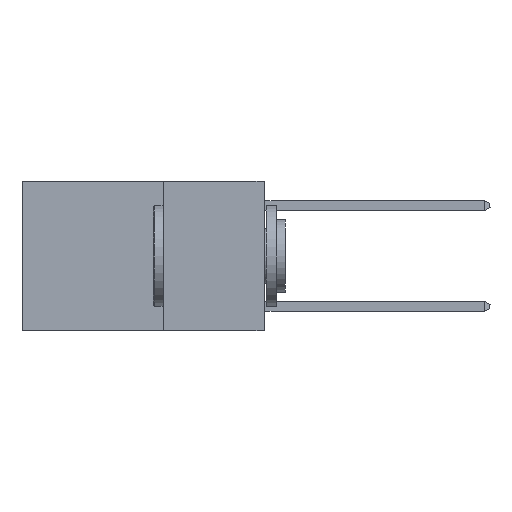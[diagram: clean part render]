
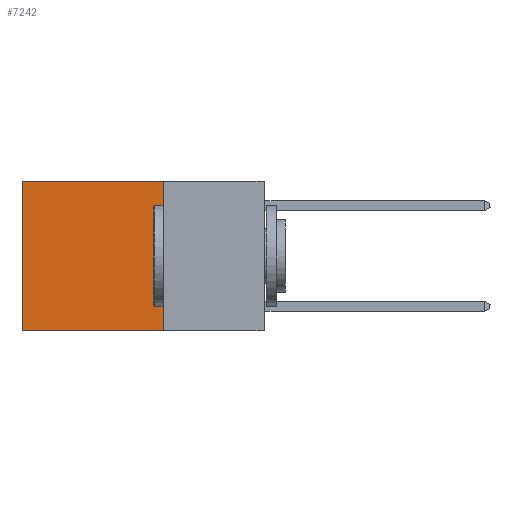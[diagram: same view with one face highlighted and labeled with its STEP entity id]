
A CAD part, left-side view. The second image highlights one B-rep face of the part: STEP entity #7242.
In plain terms, the highlighted planar face has unit normal (-1, 0, 0).
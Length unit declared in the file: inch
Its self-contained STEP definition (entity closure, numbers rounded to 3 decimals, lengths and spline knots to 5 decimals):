
#106 = CARTESIAN_POINT ( 'NONE',  ( 0.2625, 0.6, 0. ) ) ;
#512 = DIRECTION ( 'NONE',  ( 0., 1., 0. ) ) ;
#582 = VERTEX_POINT ( 'NONE', #650 ) ;
#645 = CARTESIAN_POINT ( 'NONE',  ( 0.2625, 0.25, 0. ) ) ;
#650 = CARTESIAN_POINT ( 'NONE',  ( 0.2625, 0.25, 0. ) ) ;
#1043 = VECTOR ( 'NONE', #12016, 39.37008 ) ;
#1431 = VERTEX_POINT ( 'NONE', #106 ) ;
#2022 = DIRECTION ( 'NONE',  ( 0., 0., -1. ) ) ;
#3004 = DIRECTION ( 'NONE',  ( 0., 0., -1. ) ) ;
#3962 = CARTESIAN_POINT ( 'NONE',  ( 0.2625, 0.6, 0. ) ) ;
#4202 = VECTOR ( 'NONE', #512, 39.37008 ) ;
#4542 = ORIENTED_EDGE ( 'NONE', *, *, #12662, .T. ) ;
#4945 = PLANE ( 'NONE',  #6303 ) ;
#5091 = CARTESIAN_POINT ( 'NONE',  ( 0.2625, 0.25, -0.37 ) ) ;
#5653 = VERTEX_POINT ( 'NONE', #7669 ) ;
#5945 = FACE_OUTER_BOUND ( 'NONE', #5966, .T. ) ;
#5966 = EDGE_LOOP ( 'NONE', ( #4542, #9479, #6915, #8725 ) ) ;
#6143 = LINE ( 'NONE', #5091, #1043 ) ;
#6303 = AXIS2_PLACEMENT_3D ( 'NONE', #12005, #8969, #3004 ) ;
#6915 = ORIENTED_EDGE ( 'NONE', *, *, #8393, .F. ) ;
#6950 = VECTOR ( 'NONE', #2022, 39.37008 ) ;
#7129 = LINE ( 'NONE', #3962, #6950 ) ;
#7242 = ADVANCED_FACE ( 'NONE', ( #5945 ), #4945, .F. ) ;
#7669 = CARTESIAN_POINT ( 'NONE',  ( 0.2625, 0.25, -0.37 ) ) ;
#8282 = CARTESIAN_POINT ( 'NONE',  ( 0.2625, 0.25, 0. ) ) ;
#8393 = EDGE_CURVE ( 'NONE', #582, #5653, #8728, .T. ) ;
#8725 = ORIENTED_EDGE ( 'NONE', *, *, #10030, .T. ) ;
#8728 = LINE ( 'NONE', #645, #11235 ) ;
#8969 = DIRECTION ( 'NONE',  ( 1., 0., 0. ) ) ;
#9479 = ORIENTED_EDGE ( 'NONE', *, *, #12049, .F. ) ;
#10030 = EDGE_CURVE ( 'NONE', #582, #1431, #12471, .T. ) ;
#10398 = VERTEX_POINT ( 'NONE', #12077 ) ;
#10736 = DIRECTION ( 'NONE',  ( 0., 0., -1. ) ) ;
#11235 = VECTOR ( 'NONE', #10736, 39.37008 ) ;
#12005 = CARTESIAN_POINT ( 'NONE',  ( 0.2625, 0.25, 0. ) ) ;
#12016 = DIRECTION ( 'NONE',  ( 0., 1., 0. ) ) ;
#12049 = EDGE_CURVE ( 'NONE', #5653, #10398, #6143, .T. ) ;
#12077 = CARTESIAN_POINT ( 'NONE',  ( 0.2625, 0.6, -0.37 ) ) ;
#12471 = LINE ( 'NONE', #8282, #4202 ) ;
#12662 = EDGE_CURVE ( 'NONE', #1431, #10398, #7129, .T. ) ;
